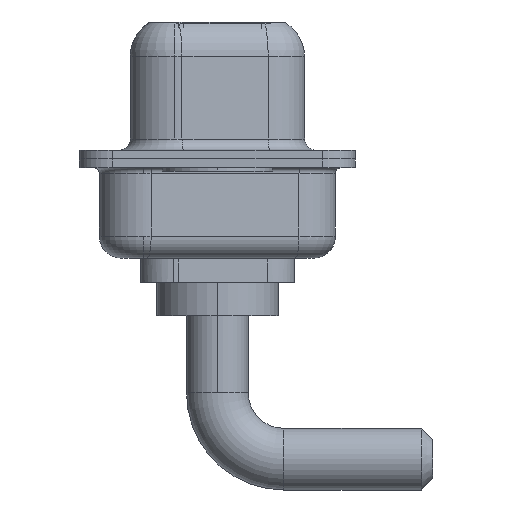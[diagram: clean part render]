
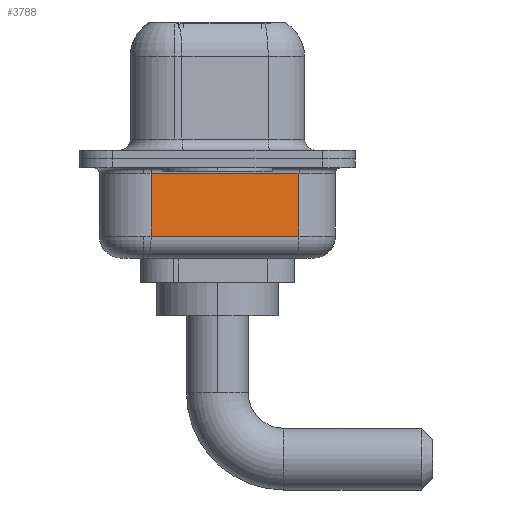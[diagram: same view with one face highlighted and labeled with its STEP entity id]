
A CAD part, left-side view. The second image highlights one B-rep face of the part: STEP entity #3788.
In plain terms, the highlighted planar face has unit normal (-0.985, -0.174, 0).
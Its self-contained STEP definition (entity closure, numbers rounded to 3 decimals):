
#197 = LINE ( 'NONE', #5419, #10285 ) ;
#1177 = VERTEX_POINT ( 'NONE', #7009 ) ;
#1413 = ORIENTED_EDGE ( 'NONE', *, *, #5797, .F. ) ;
#1430 = EDGE_CURVE ( 'NONE', #1177, #1955, #197, .T. ) ;
#1955 = VERTEX_POINT ( 'NONE', #10300 ) ;
#2542 = CARTESIAN_POINT ( 'NONE',  ( 2.88, 3.003, -3.5 ) ) ;
#2960 = VERTEX_POINT ( 'NONE', #7163 ) ;
#3288 = AXIS2_PLACEMENT_3D ( 'NONE', #10620, #7028, #9687 ) ;
#3410 = LINE ( 'NONE', #2542, #5339 ) ;
#3523 = PLANE ( 'NONE',  #3288 ) ;
#3538 = CARTESIAN_POINT ( 'NONE',  ( 2.88, 3.003, -4.5 ) ) ;
#3673 = EDGE_LOOP ( 'NONE', ( #1413, #5448, #8747, #4420 ) ) ;
#3729 = EDGE_CURVE ( 'NONE', #2960, #5310, #3410, .T. ) ;
#3788 = ADVANCED_FACE ( 'NONE', ( #9581 ), #3523, .F. ) ;
#3885 = CARTESIAN_POINT ( 'NONE',  ( 4.062, -3.697, -3.5 ) ) ;
#4353 = DIRECTION ( 'NONE',  ( 0., 0., 1. ) ) ;
#4420 = ORIENTED_EDGE ( 'NONE', *, *, #1430, .T. ) ;
#5310 = VERTEX_POINT ( 'NONE', #3885 ) ;
#5339 = VECTOR ( 'NONE', #6966, 1000. ) ;
#5419 = CARTESIAN_POINT ( 'NONE',  ( 2.88, 3.003, -0.65 ) ) ;
#5448 = ORIENTED_EDGE ( 'NONE', *, *, #3729, .T. ) ;
#5797 = EDGE_CURVE ( 'NONE', #2960, #1955, #10590, .T. ) ;
#6747 = CARTESIAN_POINT ( 'NONE',  ( 4.062, -3.697, -4.5 ) ) ;
#6966 = DIRECTION ( 'NONE',  ( 0.174, -0.985, 0. ) ) ;
#7009 = CARTESIAN_POINT ( 'NONE',  ( 4.062, -3.697, -0.65 ) ) ;
#7028 = DIRECTION ( 'NONE',  ( 0.985, 0.174, 0. ) ) ;
#7163 = CARTESIAN_POINT ( 'NONE',  ( 2.88, 3.003, -3.5 ) ) ;
#8181 = VECTOR ( 'NONE', #4353, 1000. ) ;
#8649 = VECTOR ( 'NONE', #9309, 1000. ) ;
#8747 = ORIENTED_EDGE ( 'NONE', *, *, #9271, .T. ) ;
#9271 = EDGE_CURVE ( 'NONE', #5310, #1177, #10143, .T. ) ;
#9309 = DIRECTION ( 'NONE',  ( 0., 0., 1. ) ) ;
#9581 = FACE_OUTER_BOUND ( 'NONE', #3673, .T. ) ;
#9687 = DIRECTION ( 'NONE',  ( -0.174, 0.985, 0. ) ) ;
#9897 = DIRECTION ( 'NONE',  ( -0.174, 0.985, 0. ) ) ;
#10143 = LINE ( 'NONE', #6747, #8649 ) ;
#10285 = VECTOR ( 'NONE', #9897, 1000. ) ;
#10300 = CARTESIAN_POINT ( 'NONE',  ( 2.88, 3.003, -0.65 ) ) ;
#10590 = LINE ( 'NONE', #3538, #8181 ) ;
#10620 = CARTESIAN_POINT ( 'NONE',  ( 2.88, 3.003, -4.5 ) ) ;
